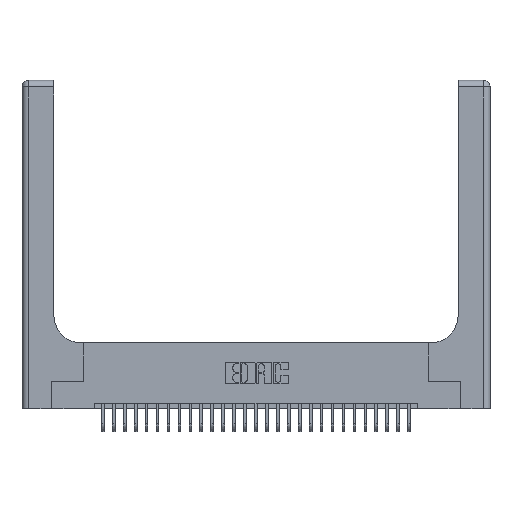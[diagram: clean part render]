
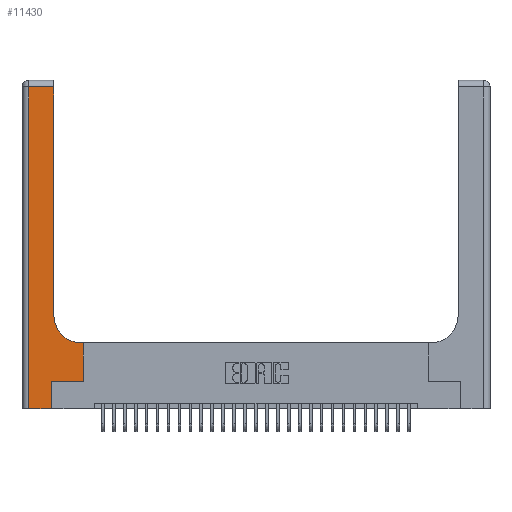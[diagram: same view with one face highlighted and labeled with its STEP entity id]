
A CAD part, top view. The second image highlights one B-rep face of the part: STEP entity #11430.
In plain terms, the highlighted planar face has unit normal (0, 0, 1).
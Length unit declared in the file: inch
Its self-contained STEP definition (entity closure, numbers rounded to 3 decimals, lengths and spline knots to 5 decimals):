
#1060 = LINE ( 'NONE', #29182, #6919 ) ;
#1508 = CARTESIAN_POINT ( 'NONE',  ( 0.2915, 2.94, 0.37 ) ) ;
#1570 = VERTEX_POINT ( 'NONE', #11295 ) ;
#1992 = VECTOR ( 'NONE', #25929, 39.37008 ) ;
#2290 = LINE ( 'NONE', #13346, #26661 ) ;
#2626 = DIRECTION ( 'NONE',  ( 0., 1., 0. ) ) ;
#2653 = ORIENTED_EDGE ( 'NONE', *, *, #10156, .T. ) ;
#3003 = EDGE_CURVE ( 'NONE', #3116, #25636, #15241, .T. ) ;
#3031 = DIRECTION ( 'NONE',  ( -1., 0., 0. ) ) ;
#3116 = VERTEX_POINT ( 'NONE', #16674 ) ;
#3921 = DIRECTION ( 'NONE',  ( -1., 0., 0. ) ) ;
#4671 = PLANE ( 'NONE',  #7925 ) ;
#4885 = EDGE_CURVE ( 'NONE', #22107, #6412, #8872, .T. ) ;
#6182 = ORIENTED_EDGE ( 'NONE', *, *, #4885, .T. ) ;
#6412 = VERTEX_POINT ( 'NONE', #15875 ) ;
#6919 = VECTOR ( 'NONE', #12504, 39.37008 ) ;
#7055 = LINE ( 'NONE', #13221, #12867 ) ;
#7368 = ORIENTED_EDGE ( 'NONE', *, *, #29152, .T. ) ;
#7744 = ORIENTED_EDGE ( 'NONE', *, *, #17085, .T. ) ;
#7925 = AXIS2_PLACEMENT_3D ( 'NONE', #12156, #28841, #14653 ) ;
#8001 = DIRECTION ( 'NONE',  ( 0., -1., 0. ) ) ;
#8872 = LINE ( 'NONE', #25817, #21781 ) ;
#9283 = ORIENTED_EDGE ( 'NONE', *, *, #12599, .T. ) ;
#10156 = EDGE_CURVE ( 'NONE', #21596, #19685, #1060, .T. ) ;
#11234 = ORIENTED_EDGE ( 'NONE', *, *, #24626, .T. ) ;
#11295 = CARTESIAN_POINT ( 'NONE',  ( 0.5415, 0.6, 0.37 ) ) ;
#11430 = ADVANCED_FACE ( 'NONE', ( #22826 ), #4671, .F. ) ;
#11594 = EDGE_LOOP ( 'NONE', ( #11234, #6182, #7744, #2653, #9283, #18132, #12377, #7368, #21827 ) ) ;
#11764 = CARTESIAN_POINT ( 'NONE',  ( 0.5415, 0.85, 0.37 ) ) ;
#11974 = CARTESIAN_POINT ( 'NONE',  ( 0.5585, 0.6, 0.37 ) ) ;
#12156 = CARTESIAN_POINT ( 'NONE',  ( 0., 3., 0.37 ) ) ;
#12377 = ORIENTED_EDGE ( 'NONE', *, *, #3003, .T. ) ;
#12504 = DIRECTION ( 'NONE',  ( 1., 0., 0. ) ) ;
#12599 = EDGE_CURVE ( 'NONE', #19685, #12901, #30808, .T. ) ;
#12628 = CARTESIAN_POINT ( 'NONE',  ( 0.269, 0., 0.37 ) ) ;
#12867 = VECTOR ( 'NONE', #25294, 39.37008 ) ;
#12901 = VERTEX_POINT ( 'NONE', #21189 ) ;
#13221 = CARTESIAN_POINT ( 'NONE',  ( 0.269, 0.25, 0.37 ) ) ;
#13346 = CARTESIAN_POINT ( 'NONE',  ( 0.2915, 3., 0.37 ) ) ;
#14237 = DIRECTION ( 'NONE',  ( 1., 0., 0. ) ) ;
#14653 = DIRECTION ( 'NONE',  ( -1., 0., 0. ) ) ;
#15241 = LINE ( 'NONE', #21173, #1992 ) ;
#15370 = AXIS2_PLACEMENT_3D ( 'NONE', #11764, #28465, #14237 ) ;
#15829 = DIRECTION ( 'NONE',  ( 0., 1., 0. ) ) ;
#15875 = CARTESIAN_POINT ( 'NONE',  ( 0.06, 2.94, 0.37 ) ) ;
#15903 = VECTOR ( 'NONE', #8001, 39.37008 ) ;
#16674 = CARTESIAN_POINT ( 'NONE',  ( 0.5585, 0.25, 0.37 ) ) ;
#16769 = LINE ( 'NONE', #24990, #28583 ) ;
#17085 = EDGE_CURVE ( 'NONE', #6412, #21596, #28456, .T. ) ;
#18132 = ORIENTED_EDGE ( 'NONE', *, *, #22681, .T. ) ;
#19301 = EDGE_CURVE ( 'NONE', #1570, #24669, #26208, .T. ) ;
#19685 = VERTEX_POINT ( 'NONE', #22921 ) ;
#20185 = CARTESIAN_POINT ( 'NONE',  ( 0.06, 3., 0.37 ) ) ;
#21173 = CARTESIAN_POINT ( 'NONE',  ( 0.5585, 0.25, 0.37 ) ) ;
#21189 = CARTESIAN_POINT ( 'NONE',  ( 0.269, 0.25, 0.37 ) ) ;
#21596 = VERTEX_POINT ( 'NONE', #31126 ) ;
#21781 = VECTOR ( 'NONE', #3921, 39.37008 ) ;
#21827 = ORIENTED_EDGE ( 'NONE', *, *, #19301, .T. ) ;
#22107 = VERTEX_POINT ( 'NONE', #1508 ) ;
#22681 = EDGE_CURVE ( 'NONE', #12901, #3116, #7055, .T. ) ;
#22826 = FACE_OUTER_BOUND ( 'NONE', #11594, .T. ) ;
#22921 = CARTESIAN_POINT ( 'NONE',  ( 0.269, 0., 0.37 ) ) ;
#23872 = VECTOR ( 'NONE', #2626, 39.37008 ) ;
#24626 = EDGE_CURVE ( 'NONE', #24669, #22107, #2290, .T. ) ;
#24669 = VERTEX_POINT ( 'NONE', #30160 ) ;
#24990 = CARTESIAN_POINT ( 'NONE',  ( 0.2915, 0.6, 0.37 ) ) ;
#25294 = DIRECTION ( 'NONE',  ( 1., 0., 0. ) ) ;
#25636 = VERTEX_POINT ( 'NONE', #11974 ) ;
#25817 = CARTESIAN_POINT ( 'NONE',  ( 0., 2.94, 0.37 ) ) ;
#25929 = DIRECTION ( 'NONE',  ( 0., 1., 0. ) ) ;
#26208 = CIRCLE ( 'NONE', #15370, 0.25 ) ;
#26661 = VECTOR ( 'NONE', #15829, 39.37008 ) ;
#28456 = LINE ( 'NONE', #20185, #15903 ) ;
#28465 = DIRECTION ( 'NONE',  ( 0., 0., -1. ) ) ;
#28583 = VECTOR ( 'NONE', #3031, 39.37008 ) ;
#28841 = DIRECTION ( 'NONE',  ( 0., 0., -1. ) ) ;
#29152 = EDGE_CURVE ( 'NONE', #25636, #1570, #16769, .T. ) ;
#29182 = CARTESIAN_POINT ( 'NONE',  ( 0., 0., 0.37 ) ) ;
#30160 = CARTESIAN_POINT ( 'NONE',  ( 0.2915, 0.85, 0.37 ) ) ;
#30808 = LINE ( 'NONE', #12628, #23872 ) ;
#31126 = CARTESIAN_POINT ( 'NONE',  ( 0.06, 0., 0.37 ) ) ;
